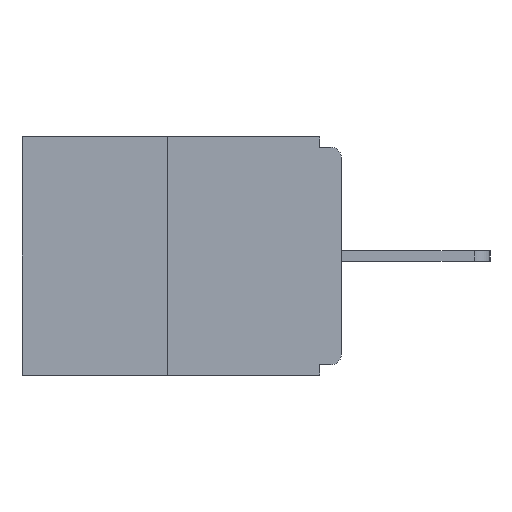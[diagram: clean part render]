
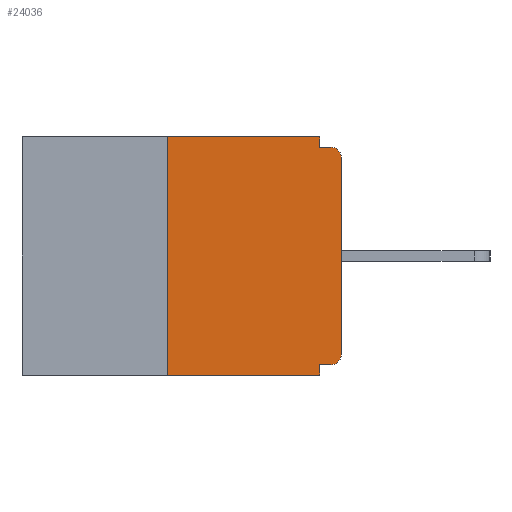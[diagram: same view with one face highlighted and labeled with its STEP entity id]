
A CAD part, left-side view. The second image highlights one B-rep face of the part: STEP entity #24036.
In plain terms, the highlighted planar face has unit normal (-1, 0, 0).
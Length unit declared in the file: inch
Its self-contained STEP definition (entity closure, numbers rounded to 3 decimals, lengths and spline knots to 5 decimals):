
#399 = CARTESIAN_POINT ( 'NONE',  ( 0., 0.25, -0.343 ) ) ;
#544 = VERTEX_POINT ( 'NONE', #23225 ) ;
#802 = DIRECTION ( 'NONE',  ( 0., -1., 0. ) ) ;
#1686 = VECTOR ( 'NONE', #16859, 39.37008 ) ;
#2014 = DIRECTION ( 'NONE',  ( 0., 0., -1. ) ) ;
#2119 = CARTESIAN_POINT ( 'NONE',  ( 0., 0.015, -0.03 ) ) ;
#2678 = VECTOR ( 'NONE', #10386, 39.37008 ) ;
#2690 = EDGE_CURVE ( 'NONE', #18254, #3167, #14286, .T. ) ;
#2723 = EDGE_CURVE ( 'NONE', #544, #16631, #26708, .T. ) ;
#2882 = VERTEX_POINT ( 'NONE', #3045 ) ;
#3045 = CARTESIAN_POINT ( 'NONE',  ( 0., 0., -0.03 ) ) ;
#3167 = VERTEX_POINT ( 'NONE', #25547 ) ;
#3785 = EDGE_CURVE ( 'NONE', #22504, #18254, #6458, .T. ) ;
#4913 = CARTESIAN_POINT ( 'NONE',  ( 0., 0.015, -0.313 ) ) ;
#5010 = EDGE_CURVE ( 'NONE', #23881, #3167, #18202, .T. ) ;
#5043 = VECTOR ( 'NONE', #10257, 39.37008 ) ;
#5177 = DIRECTION ( 'NONE',  ( -1., 0., 0. ) ) ;
#5244 = PLANE ( 'NONE',  #9526 ) ;
#5520 = CARTESIAN_POINT ( 'NONE',  ( 0., 0.031, 0. ) ) ;
#5879 = VERTEX_POINT ( 'NONE', #9743 ) ;
#5974 = EDGE_LOOP ( 'NONE', ( #6998, #24663, #11805, #14916, #20325, #26184, #13662, #25504, #25018, #19920 ) ) ;
#6397 = CIRCLE ( 'NONE', #15003, 0.015 ) ;
#6458 = LINE ( 'NONE', #14557, #2678 ) ;
#6998 = ORIENTED_EDGE ( 'NONE', *, *, #22545, .F. ) ;
#7965 = DIRECTION ( 'NONE',  ( 0., -1., 0. ) ) ;
#8117 = CARTESIAN_POINT ( 'NONE',  ( 0., 0., -0.015 ) ) ;
#8649 = LINE ( 'NONE', #10140, #1686 ) ;
#8890 = CARTESIAN_POINT ( 'NONE',  ( 0., 0.46, 0. ) ) ;
#9526 = AXIS2_PLACEMENT_3D ( 'NONE', #9691, #13477, #17906 ) ;
#9691 = CARTESIAN_POINT ( 'NONE',  ( 0., 0.46, 0. ) ) ;
#9714 = CARTESIAN_POINT ( 'NONE',  ( 0., 0.031, -0.343 ) ) ;
#9743 = CARTESIAN_POINT ( 'NONE',  ( 0., 0.25, 0. ) ) ;
#10140 = CARTESIAN_POINT ( 'NONE',  ( 0., 0.25, 0. ) ) ;
#10257 = DIRECTION ( 'NONE',  ( 0., 0., -1. ) ) ;
#10386 = DIRECTION ( 'NONE',  ( 0., 1., 0. ) ) ;
#10816 = VERTEX_POINT ( 'NONE', #26206 ) ;
#11121 = DIRECTION ( 'NONE',  ( 0., 0., -1. ) ) ;
#11450 = LINE ( 'NONE', #23874, #12843 ) ;
#11805 = ORIENTED_EDGE ( 'NONE', *, *, #5010, .T. ) ;
#12843 = VECTOR ( 'NONE', #13589, 39.37008 ) ;
#13477 = DIRECTION ( 'NONE',  ( 1., 0., 0. ) ) ;
#13589 = DIRECTION ( 'NONE',  ( 0., 0., 1. ) ) ;
#13662 = ORIENTED_EDGE ( 'NONE', *, *, #13961, .T. ) ;
#13725 = FACE_OUTER_BOUND ( 'NONE', #5974, .T. ) ;
#13961 = EDGE_CURVE ( 'NONE', #10816, #2882, #11450, .T. ) ;
#14055 = EDGE_CURVE ( 'NONE', #2882, #19881, #26619, .T. ) ;
#14286 = LINE ( 'NONE', #9714, #16675 ) ;
#14557 = CARTESIAN_POINT ( 'NONE',  ( 0., 0., -0.328 ) ) ;
#14916 = ORIENTED_EDGE ( 'NONE', *, *, #2690, .F. ) ;
#14960 = LINE ( 'NONE', #8890, #17112 ) ;
#15003 = AXIS2_PLACEMENT_3D ( 'NONE', #4913, #5177, #11121 ) ;
#16027 = CARTESIAN_POINT ( 'NONE',  ( 0., 0.031, -0.328 ) ) ;
#16127 = EDGE_CURVE ( 'NONE', #22504, #10816, #6397, .T. ) ;
#16631 = VERTEX_POINT ( 'NONE', #22650 ) ;
#16675 = VECTOR ( 'NONE', #2014, 39.37008 ) ;
#16751 = VECTOR ( 'NONE', #22563, 39.37008 ) ;
#16859 = DIRECTION ( 'NONE',  ( 0., 0., 1. ) ) ;
#17112 = VECTOR ( 'NONE', #802, 39.37008 ) ;
#17906 = DIRECTION ( 'NONE',  ( 0., 0., -1. ) ) ;
#17964 = EDGE_CURVE ( 'NONE', #23881, #5879, #8649, .T. ) ;
#17972 = EDGE_CURVE ( 'NONE', #16631, #19881, #18352, .T. ) ;
#18063 = CARTESIAN_POINT ( 'NONE',  ( 0., 0.46, -0.343 ) ) ;
#18202 = LINE ( 'NONE', #18063, #18444 ) ;
#18254 = VERTEX_POINT ( 'NONE', #16027 ) ;
#18313 = CARTESIAN_POINT ( 'NONE',  ( 0., 0.015, -0.328 ) ) ;
#18352 = LINE ( 'NONE', #8117, #16751 ) ;
#18444 = VECTOR ( 'NONE', #7965, 39.37008 ) ;
#18579 = DIRECTION ( 'NONE',  ( 0., 0., -1. ) ) ;
#19881 = VERTEX_POINT ( 'NONE', #23005 ) ;
#19920 = ORIENTED_EDGE ( 'NONE', *, *, #2723, .F. ) ;
#20325 = ORIENTED_EDGE ( 'NONE', *, *, #3785, .F. ) ;
#22504 = VERTEX_POINT ( 'NONE', #18313 ) ;
#22545 = EDGE_CURVE ( 'NONE', #5879, #544, #14960, .T. ) ;
#22563 = DIRECTION ( 'NONE',  ( 0., -1., 0. ) ) ;
#22650 = CARTESIAN_POINT ( 'NONE',  ( 0., 0.031, -0.015 ) ) ;
#22770 = AXIS2_PLACEMENT_3D ( 'NONE', #2119, #26535, #18579 ) ;
#23005 = CARTESIAN_POINT ( 'NONE',  ( 0., 0.015, -0.015 ) ) ;
#23225 = CARTESIAN_POINT ( 'NONE',  ( 0., 0.031, 0. ) ) ;
#23874 = CARTESIAN_POINT ( 'NONE',  ( 0., 0., 0. ) ) ;
#23881 = VERTEX_POINT ( 'NONE', #399 ) ;
#24036 = ADVANCED_FACE ( 'NONE', ( #13725 ), #5244, .F. ) ;
#24663 = ORIENTED_EDGE ( 'NONE', *, *, #17964, .F. ) ;
#25018 = ORIENTED_EDGE ( 'NONE', *, *, #17972, .F. ) ;
#25504 = ORIENTED_EDGE ( 'NONE', *, *, #14055, .T. ) ;
#25547 = CARTESIAN_POINT ( 'NONE',  ( 0., 0.031, -0.343 ) ) ;
#26184 = ORIENTED_EDGE ( 'NONE', *, *, #16127, .T. ) ;
#26206 = CARTESIAN_POINT ( 'NONE',  ( 0., 0., -0.313 ) ) ;
#26535 = DIRECTION ( 'NONE',  ( -1., 0., 0. ) ) ;
#26619 = CIRCLE ( 'NONE', #22770, 0.015 ) ;
#26708 = LINE ( 'NONE', #5520, #5043 ) ;
